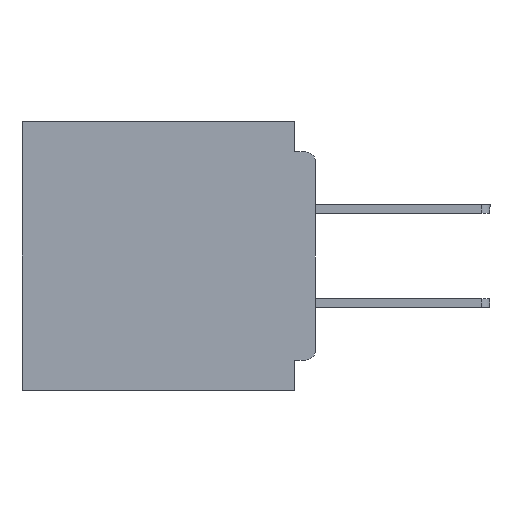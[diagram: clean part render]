
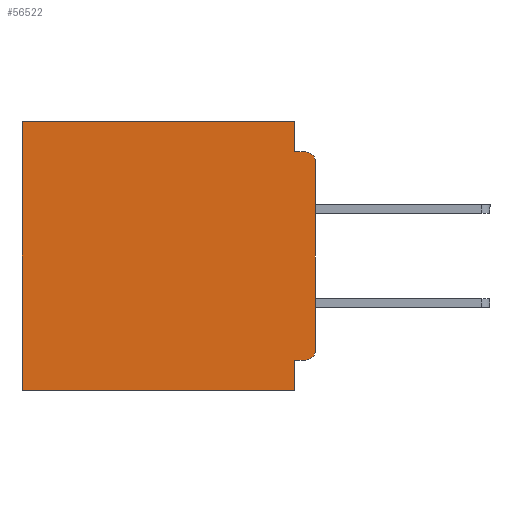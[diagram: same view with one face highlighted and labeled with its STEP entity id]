
A CAD part, left-side view. The second image highlights one B-rep face of the part: STEP entity #56522.
In plain terms, the highlighted planar face has unit normal (-1, 0, 0).
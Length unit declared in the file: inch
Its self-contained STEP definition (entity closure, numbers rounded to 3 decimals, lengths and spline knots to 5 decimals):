
#111 = DIRECTION ( 'NONE',  ( 0., 0., -1. ) ) ;
#176 = PLANE ( 'NONE',  #1251 ) ;
#1142 = EDGE_CURVE ( 'NONE', #25561, #20694, #18892, .T. ) ;
#1251 = AXIS2_PLACEMENT_3D ( 'NONE', #38792, #4634, #35537 ) ;
#1344 = VECTOR ( 'NONE', #54987, 39.37008 ) ;
#2300 = DIRECTION ( 'NONE',  ( 0., 0., -1. ) ) ;
#2377 = LINE ( 'NONE', #13365, #14194 ) ;
#2911 = LINE ( 'NONE', #27556, #47000 ) ;
#4007 = CARTESIAN_POINT ( 'NONE',  ( 0.3, 0.015, -0.045 ) ) ;
#4634 = DIRECTION ( 'NONE',  ( 1., 0., 0. ) ) ;
#4859 = VERTEX_POINT ( 'NONE', #48319 ) ;
#6160 = CARTESIAN_POINT ( 'NONE',  ( 0.3, 0., -0.045 ) ) ;
#6419 = CARTESIAN_POINT ( 'NONE',  ( 0.3, 0., 0. ) ) ;
#8924 = EDGE_CURVE ( 'NONE', #38827, #9514, #22886, .T. ) ;
#9514 = VERTEX_POINT ( 'NONE', #51110 ) ;
#9928 = LINE ( 'NONE', #41918, #32029 ) ;
#9934 = DIRECTION ( 'NONE',  ( 0., -1., 0. ) ) ;
#12895 = EDGE_CURVE ( 'NONE', #39052, #45297, #2911, .T. ) ;
#13365 = CARTESIAN_POINT ( 'NONE',  ( 0.3, 0.031, 0. ) ) ;
#14194 = VECTOR ( 'NONE', #111, 39.37008 ) ;
#14241 = ORIENTED_EDGE ( 'NONE', *, *, #8924, .F. ) ;
#15124 = AXIS2_PLACEMENT_3D ( 'NONE', #51248, #25153, #55646 ) ;
#15684 = CARTESIAN_POINT ( 'NONE',  ( 0.3, 0.437, -0.4 ) ) ;
#16168 = CARTESIAN_POINT ( 'NONE',  ( 0.3, 0., -0.4 ) ) ;
#16182 = CARTESIAN_POINT ( 'NONE',  ( 0.3, 0., -0.06 ) ) ;
#17372 = ORIENTED_EDGE ( 'NONE', *, *, #47332, .T. ) ;
#18887 = DIRECTION ( 'NONE',  ( 0., 0., -1. ) ) ;
#18892 = LINE ( 'NONE', #6160, #51046 ) ;
#19046 = VERTEX_POINT ( 'NONE', #36729 ) ;
#19818 = EDGE_CURVE ( 'NONE', #23941, #39052, #44091, .T. ) ;
#20694 = VERTEX_POINT ( 'NONE', #4007 ) ;
#20822 = VECTOR ( 'NONE', #33064, 39.37008 ) ;
#22275 = EDGE_CURVE ( 'NONE', #23941, #25561, #2377, .T. ) ;
#22535 = ORIENTED_EDGE ( 'NONE', *, *, #23891, .F. ) ;
#22886 = LINE ( 'NONE', #24487, #37184 ) ;
#23891 = EDGE_CURVE ( 'NONE', #19046, #38827, #9928, .T. ) ;
#23941 = VERTEX_POINT ( 'NONE', #38069 ) ;
#24099 = CARTESIAN_POINT ( 'NONE',  ( 0.3, 0.031, -0.355 ) ) ;
#24487 = CARTESIAN_POINT ( 'NONE',  ( 0.3, 0.031, -0.4 ) ) ;
#24497 = CARTESIAN_POINT ( 'NONE',  ( 0.3, 0., -0.4 ) ) ;
#24617 = DIRECTION ( 'NONE',  ( -1., 0., 0. ) ) ;
#25153 = DIRECTION ( 'NONE',  ( -1., 0., 0. ) ) ;
#25242 = CIRCLE ( 'NONE', #15124, 0.015 ) ;
#25561 = VERTEX_POINT ( 'NONE', #40973 ) ;
#25787 = EDGE_CURVE ( 'NONE', #19046, #4859, #25242, .T. ) ;
#27556 = CARTESIAN_POINT ( 'NONE',  ( 0.3, 0.437, -0.4 ) ) ;
#28933 = DIRECTION ( 'NONE',  ( 0., 1., 0. ) ) ;
#29418 = VERTEX_POINT ( 'NONE', #16182 ) ;
#30932 = AXIS2_PLACEMENT_3D ( 'NONE', #50716, #24617, #55116 ) ;
#32029 = VECTOR ( 'NONE', #28933, 39.37008 ) ;
#32878 = FACE_OUTER_BOUND ( 'NONE', #49067, .T. ) ;
#33064 = DIRECTION ( 'NONE',  ( 0., 1., 0. ) ) ;
#33672 = CIRCLE ( 'NONE', #30932, 0.015 ) ;
#33841 = DIRECTION ( 'NONE',  ( 0., 1., 0. ) ) ;
#34174 = CARTESIAN_POINT ( 'NONE',  ( 0.3, 0.437, 0. ) ) ;
#34770 = EDGE_CURVE ( 'NONE', #9514, #45297, #37705, .T. ) ;
#35229 = LINE ( 'NONE', #24497, #1344 ) ;
#35537 = DIRECTION ( 'NONE',  ( 0., 0., -1. ) ) ;
#36729 = CARTESIAN_POINT ( 'NONE',  ( 0.3, 0.015, -0.355 ) ) ;
#37184 = VECTOR ( 'NONE', #2300, 39.37008 ) ;
#37705 = LINE ( 'NONE', #16168, #46606 ) ;
#38069 = CARTESIAN_POINT ( 'NONE',  ( 0.3, 0.031, 0. ) ) ;
#38453 = ORIENTED_EDGE ( 'NONE', *, *, #19818, .T. ) ;
#38792 = CARTESIAN_POINT ( 'NONE',  ( 0.3, 0., -0.4 ) ) ;
#38827 = VERTEX_POINT ( 'NONE', #24099 ) ;
#38879 = EDGE_CURVE ( 'NONE', #29418, #4859, #35229, .T. ) ;
#39052 = VERTEX_POINT ( 'NONE', #34174 ) ;
#39094 = ORIENTED_EDGE ( 'NONE', *, *, #34770, .F. ) ;
#40973 = CARTESIAN_POINT ( 'NONE',  ( 0.3, 0.031, -0.045 ) ) ;
#41918 = CARTESIAN_POINT ( 'NONE',  ( 0.3, 0., -0.355 ) ) ;
#44091 = LINE ( 'NONE', #6419, #20822 ) ;
#44533 = ORIENTED_EDGE ( 'NONE', *, *, #22275, .F. ) ;
#45297 = VERTEX_POINT ( 'NONE', #15684 ) ;
#46606 = VECTOR ( 'NONE', #33841, 39.37008 ) ;
#47000 = VECTOR ( 'NONE', #18887, 39.37008 ) ;
#47332 = EDGE_CURVE ( 'NONE', #29418, #20694, #33672, .T. ) ;
#48319 = CARTESIAN_POINT ( 'NONE',  ( 0.3, 0., -0.34 ) ) ;
#48563 = ORIENTED_EDGE ( 'NONE', *, *, #12895, .T. ) ;
#49015 = ORIENTED_EDGE ( 'NONE', *, *, #38879, .F. ) ;
#49053 = ORIENTED_EDGE ( 'NONE', *, *, #25787, .T. ) ;
#49067 = EDGE_LOOP ( 'NONE', ( #49015, #17372, #52025, #44533, #38453, #48563, #39094, #14241, #22535, #49053 ) ) ;
#50716 = CARTESIAN_POINT ( 'NONE',  ( 0.3, 0.015, -0.06 ) ) ;
#51046 = VECTOR ( 'NONE', #9934, 39.37008 ) ;
#51110 = CARTESIAN_POINT ( 'NONE',  ( 0.3, 0.031, -0.4 ) ) ;
#51248 = CARTESIAN_POINT ( 'NONE',  ( 0.3, 0.015, -0.34 ) ) ;
#52025 = ORIENTED_EDGE ( 'NONE', *, *, #1142, .F. ) ;
#54987 = DIRECTION ( 'NONE',  ( 0., 0., -1. ) ) ;
#55116 = DIRECTION ( 'NONE',  ( 0., 0., -1. ) ) ;
#55646 = DIRECTION ( 'NONE',  ( 0., 0., -1. ) ) ;
#56522 = ADVANCED_FACE ( 'NONE', ( #32878 ), #176, .F. ) ;
